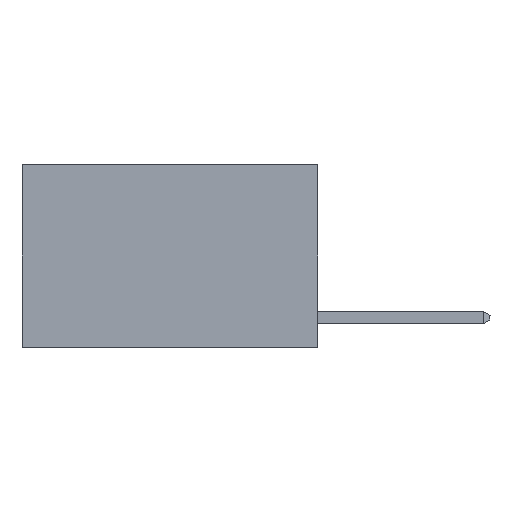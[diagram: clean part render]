
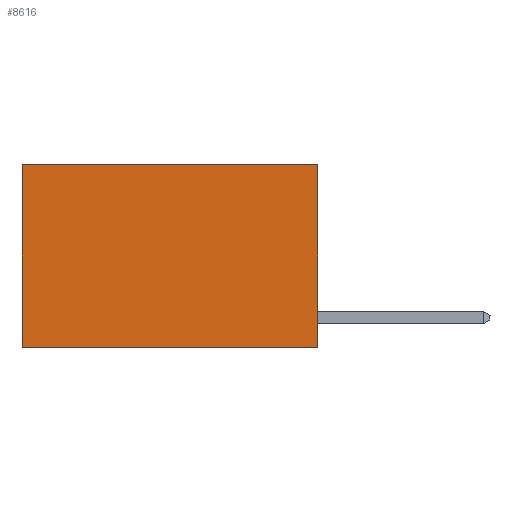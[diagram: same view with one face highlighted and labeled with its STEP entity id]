
A CAD part, left-side view. The second image highlights one B-rep face of the part: STEP entity #8616.
In plain terms, the highlighted planar face has unit normal (-1, 0, 0).
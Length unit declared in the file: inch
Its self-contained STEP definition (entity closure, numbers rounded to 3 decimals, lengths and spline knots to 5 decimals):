
#195 = ORIENTED_EDGE ( 'NONE', *, *, #8814, .T. ) ;
#199 = CARTESIAN_POINT ( 'NONE',  ( 0.2625, 0., -0.37 ) ) ;
#530 = DIRECTION ( 'NONE',  ( 1., 0., 0. ) ) ;
#1027 = DIRECTION ( 'NONE',  ( 0., 1., 0. ) ) ;
#1144 = CARTESIAN_POINT ( 'NONE',  ( 0.2625, 0., -0.37 ) ) ;
#1210 = VECTOR ( 'NONE', #1027, 39.37008 ) ;
#1721 = VERTEX_POINT ( 'NONE', #1144 ) ;
#1928 = DIRECTION ( 'NONE',  ( 0., 0., -1. ) ) ;
#1965 = CARTESIAN_POINT ( 'NONE',  ( 0.2625, 0., 0. ) ) ;
#2947 = CARTESIAN_POINT ( 'NONE',  ( 0.2625, 0.6, 0. ) ) ;
#3151 = FACE_OUTER_BOUND ( 'NONE', #5121, .T. ) ;
#4302 = ORIENTED_EDGE ( 'NONE', *, *, #9738, .F. ) ;
#4740 = CARTESIAN_POINT ( 'NONE',  ( 0.2625, 0.6, 0. ) ) ;
#4759 = EDGE_CURVE ( 'NONE', #1721, #10932, #11955, .T. ) ;
#5121 = EDGE_LOOP ( 'NONE', ( #14424, #14658, #4302, #195 ) ) ;
#5837 = CARTESIAN_POINT ( 'NONE',  ( 0.2625, 0., 0. ) ) ;
#5888 = EDGE_CURVE ( 'NONE', #13431, #10932, #13352, .T. ) ;
#7561 = CARTESIAN_POINT ( 'NONE',  ( 0.2625, 0.6, -0.37 ) ) ;
#8064 = DIRECTION ( 'NONE',  ( 0., 0., -1. ) ) ;
#8421 = CARTESIAN_POINT ( 'NONE',  ( 0.2625, 0., 0. ) ) ;
#8517 = VECTOR ( 'NONE', #13062, 39.37008 ) ;
#8616 = ADVANCED_FACE ( 'NONE', ( #3151 ), #10694, .F. ) ;
#8814 = EDGE_CURVE ( 'NONE', #9976, #13431, #13785, .T. ) ;
#9457 = VECTOR ( 'NONE', #8064, 39.37008 ) ;
#9729 = LINE ( 'NONE', #11081, #10304 ) ;
#9738 = EDGE_CURVE ( 'NONE', #9976, #1721, #9729, .T. ) ;
#9976 = VERTEX_POINT ( 'NONE', #5837 ) ;
#10304 = VECTOR ( 'NONE', #1928, 39.37008 ) ;
#10598 = AXIS2_PLACEMENT_3D ( 'NONE', #1965, #530, #10867 ) ;
#10694 = PLANE ( 'NONE',  #10598 ) ;
#10867 = DIRECTION ( 'NONE',  ( 0., 0., -1. ) ) ;
#10932 = VERTEX_POINT ( 'NONE', #7561 ) ;
#11081 = CARTESIAN_POINT ( 'NONE',  ( 0.2625, 0., 0. ) ) ;
#11955 = LINE ( 'NONE', #199, #8517 ) ;
#13062 = DIRECTION ( 'NONE',  ( 0., 1., 0. ) ) ;
#13352 = LINE ( 'NONE', #2947, #9457 ) ;
#13431 = VERTEX_POINT ( 'NONE', #4740 ) ;
#13785 = LINE ( 'NONE', #8421, #1210 ) ;
#14424 = ORIENTED_EDGE ( 'NONE', *, *, #5888, .T. ) ;
#14658 = ORIENTED_EDGE ( 'NONE', *, *, #4759, .F. ) ;
